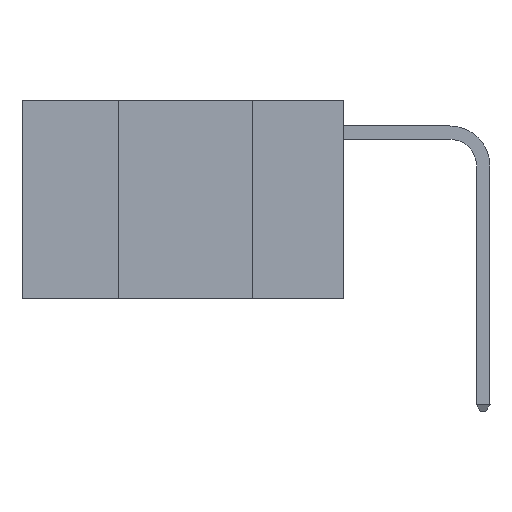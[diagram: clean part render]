
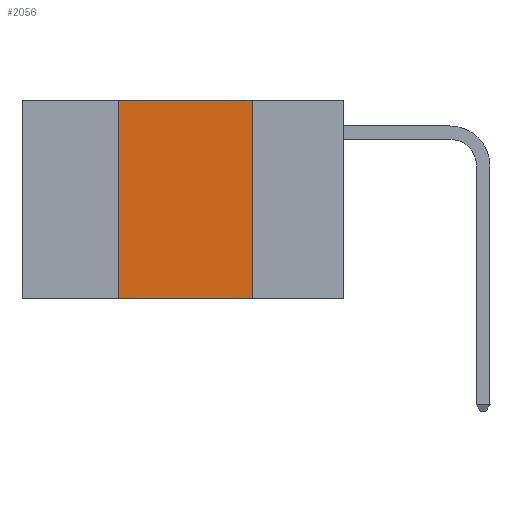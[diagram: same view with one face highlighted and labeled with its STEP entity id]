
A CAD part, left-side view. The second image highlights one B-rep face of the part: STEP entity #2056.
In plain terms, the highlighted planar face has unit normal (-1, 0, 0).
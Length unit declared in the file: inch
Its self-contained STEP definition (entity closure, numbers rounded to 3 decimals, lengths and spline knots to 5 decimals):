
#79 = VECTOR ( 'NONE', #13903, 39.37008 ) ;
#762 = CARTESIAN_POINT ( 'NONE',  ( 0., 0.6, -0.37 ) ) ;
#1001 = DIRECTION ( 'NONE',  ( 0., 0., 1. ) ) ;
#1649 = CARTESIAN_POINT ( 'NONE',  ( 0., 0.17, 0. ) ) ;
#1946 = EDGE_CURVE ( 'NONE', #3920, #7691, #21637, .T. ) ;
#2056 = ADVANCED_FACE ( 'NONE', ( #24373 ), #24447, .F. ) ;
#2264 = CARTESIAN_POINT ( 'NONE',  ( 0., 0.17, 0. ) ) ;
#3105 = DIRECTION ( 'NONE',  ( 0., 0., -1. ) ) ;
#3920 = VERTEX_POINT ( 'NONE', #17824 ) ;
#4839 = ORIENTED_EDGE ( 'NONE', *, *, #11047, .F. ) ;
#5012 = LINE ( 'NONE', #1649, #9586 ) ;
#6937 = CARTESIAN_POINT ( 'NONE',  ( 0., 0.42, 0. ) ) ;
#7691 = VERTEX_POINT ( 'NONE', #9745 ) ;
#9386 = AXIS2_PLACEMENT_3D ( 'NONE', #12839, #14826, #3105 ) ;
#9586 = VECTOR ( 'NONE', #21042, 39.37008 ) ;
#9745 = CARTESIAN_POINT ( 'NONE',  ( 0., 0.17, -0.37 ) ) ;
#9810 = ORIENTED_EDGE ( 'NONE', *, *, #21079, .F. ) ;
#10593 = VERTEX_POINT ( 'NONE', #2264 ) ;
#11047 = EDGE_CURVE ( 'NONE', #10593, #7691, #5012, .T. ) ;
#11334 = VECTOR ( 'NONE', #12507, 39.37008 ) ;
#12507 = DIRECTION ( 'NONE',  ( 0., -1., 0. ) ) ;
#12839 = CARTESIAN_POINT ( 'NONE',  ( 0., 0.6, 0. ) ) ;
#13373 = VECTOR ( 'NONE', #1001, 39.37008 ) ;
#13384 = EDGE_LOOP ( 'NONE', ( #4839, #9810, #15611, #18261 ) ) ;
#13579 = CARTESIAN_POINT ( 'NONE',  ( 0., 0.42, 0. ) ) ;
#13715 = EDGE_CURVE ( 'NONE', #3920, #20436, #23673, .T. ) ;
#13903 = DIRECTION ( 'NONE',  ( 0., -1., 0. ) ) ;
#14826 = DIRECTION ( 'NONE',  ( 1., 0., 0. ) ) ;
#15611 = ORIENTED_EDGE ( 'NONE', *, *, #13715, .F. ) ;
#17824 = CARTESIAN_POINT ( 'NONE',  ( 0., 0.42, -0.37 ) ) ;
#18261 = ORIENTED_EDGE ( 'NONE', *, *, #1946, .T. ) ;
#20436 = VERTEX_POINT ( 'NONE', #13579 ) ;
#21042 = DIRECTION ( 'NONE',  ( 0., 0., -1. ) ) ;
#21079 = EDGE_CURVE ( 'NONE', #20436, #10593, #24820, .T. ) ;
#21637 = LINE ( 'NONE', #762, #11334 ) ;
#23541 = CARTESIAN_POINT ( 'NONE',  ( 0., 0.6, 0. ) ) ;
#23673 = LINE ( 'NONE', #6937, #13373 ) ;
#24373 = FACE_OUTER_BOUND ( 'NONE', #13384, .T. ) ;
#24447 = PLANE ( 'NONE',  #9386 ) ;
#24820 = LINE ( 'NONE', #23541, #79 ) ;
